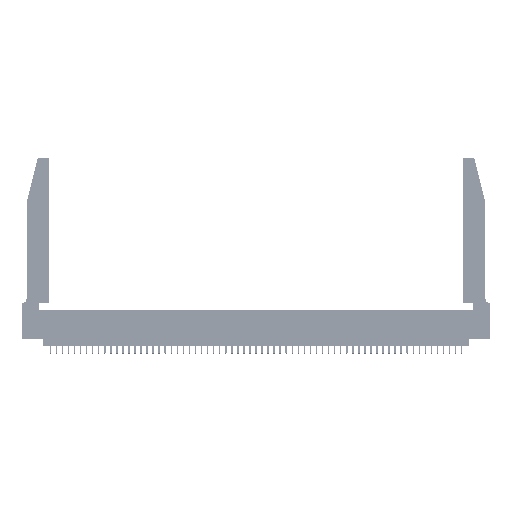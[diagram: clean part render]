
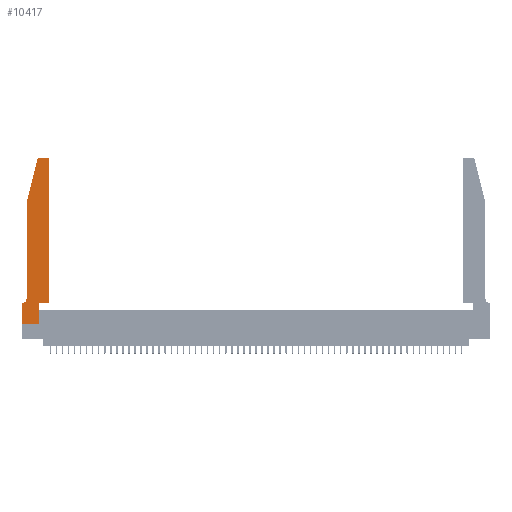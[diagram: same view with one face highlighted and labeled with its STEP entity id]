
A CAD part, top view. The second image highlights one B-rep face of the part: STEP entity #10417.
In plain terms, the highlighted planar face has unit normal (0, 0, 1).
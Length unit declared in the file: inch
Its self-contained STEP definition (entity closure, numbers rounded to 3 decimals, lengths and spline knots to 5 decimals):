
#891 = PLANE ( 'NONE',  #10989 ) ;
#2058 = EDGE_CURVE ( 'NONE', #8931, #30451, #37048, .T. ) ;
#2872 = DIRECTION ( 'NONE',  ( 0., 1., 0. ) ) ;
#3348 = ORIENTED_EDGE ( 'NONE', *, *, #26619, .T. ) ;
#3989 = CARTESIAN_POINT ( 'NONE',  ( 0.4205, 2.75, 0.37 ) ) ;
#4264 = AXIS2_PLACEMENT_3D ( 'NONE', #21716, #38909, #36018 ) ;
#4427 = EDGE_CURVE ( 'NONE', #45194, #24792, #38880, .T. ) ;
#4433 = VECTOR ( 'NONE', #43023, 39.37008 ) ;
#4806 = DIRECTION ( 'NONE',  ( 0., 0., 1. ) ) ;
#4918 = CARTESIAN_POINT ( 'NONE',  ( 0.4505, 0.35, 0.37 ) ) ;
#6414 = ORIENTED_EDGE ( 'NONE', *, *, #10900, .T. ) ;
#8605 = CARTESIAN_POINT ( 'NONE',  ( 0., 0.35, 0.37 ) ) ;
#8931 = VERTEX_POINT ( 'NONE', #50287 ) ;
#9061 = EDGE_CURVE ( 'NONE', #31428, #45194, #43631, .T. ) ;
#9424 = CARTESIAN_POINT ( 'NONE',  ( 0.4505, 0.35, 0.37 ) ) ;
#10417 = ADVANCED_FACE ( 'NONE', ( #13896 ), #891, .T. ) ;
#10900 = EDGE_CURVE ( 'NONE', #27365, #42193, #46105, .T. ) ;
#10989 = AXIS2_PLACEMENT_3D ( 'NONE', #25953, #4806, #17506 ) ;
#12014 = EDGE_CURVE ( 'NONE', #42193, #31428, #12374, .T. ) ;
#12374 = LINE ( 'NONE', #21118, #4433 ) ;
#12506 = LINE ( 'NONE', #4918, #15185 ) ;
#12856 = AXIS2_PLACEMENT_3D ( 'NONE', #47178, #42921, #17224 ) ;
#13137 = EDGE_CURVE ( 'NONE', #27929, #8931, #24853, .T. ) ;
#13896 = FACE_OUTER_BOUND ( 'NONE', #14380, .T. ) ;
#14380 = EDGE_LOOP ( 'NONE', ( #22211, #6414, #25425, #33420, #42155, #39651, #44276, #36805, #36044, #3348, #30424, #37566 ) ) ;
#14852 = VECTOR ( 'NONE', #47468, 39.37008 ) ;
#15185 = VECTOR ( 'NONE', #34869, 39.37008 ) ;
#17224 = DIRECTION ( 'NONE',  ( 1., 0., 0. ) ) ;
#17421 = CARTESIAN_POINT ( 'NONE',  ( 0.2865, 0.35, 0.37 ) ) ;
#17432 = LINE ( 'NONE', #52003, #25488 ) ;
#17506 = DIRECTION ( 'NONE',  ( 1., 0., 0. ) ) ;
#17520 = CARTESIAN_POINT ( 'NONE',  ( 0.2865, 0.35, 0.37 ) ) ;
#17792 = CARTESIAN_POINT ( 'NONE',  ( 0., 0., 0.37 ) ) ;
#18248 = EDGE_CURVE ( 'NONE', #48415, #41731, #26283, .T. ) ;
#19360 = CARTESIAN_POINT ( 'NONE',  ( 0.0755, 2., 0.37 ) ) ;
#21118 = CARTESIAN_POINT ( 'NONE',  ( 0.0755, 2., 0.37 ) ) ;
#21716 = CARTESIAN_POINT ( 'NONE',  ( 0.284, 2.72, 0.37 ) ) ;
#22126 = DIRECTION ( 'NONE',  ( 0., -1., 0. ) ) ;
#22211 = ORIENTED_EDGE ( 'NONE', *, *, #51842, .T. ) ;
#22424 = CARTESIAN_POINT ( 'NONE',  ( 0.284, 2.75, 0.37 ) ) ;
#23789 = DIRECTION ( 'NONE',  ( 0., 0., -1. ) ) ;
#23941 = DIRECTION ( 'NONE',  ( -1., 0., 0. ) ) ;
#24792 = VERTEX_POINT ( 'NONE', #25930 ) ;
#24811 = CARTESIAN_POINT ( 'NONE',  ( 0., 0., 0.37 ) ) ;
#24853 = LINE ( 'NONE', #50204, #46906 ) ;
#25425 = ORIENTED_EDGE ( 'NONE', *, *, #12014, .T. ) ;
#25488 = VECTOR ( 'NONE', #29948, 39.37008 ) ;
#25910 = DIRECTION ( 'NONE',  ( 0., -1., 0. ) ) ;
#25930 = CARTESIAN_POINT ( 'NONE',  ( 0.0055, 0.35, 0.37 ) ) ;
#25953 = CARTESIAN_POINT ( 'NONE',  ( 0., 0.35, 0.37 ) ) ;
#26283 = LINE ( 'NONE', #17520, #14852 ) ;
#26349 = CARTESIAN_POINT ( 'NONE',  ( 0.25487, 2.72718, 0.37 ) ) ;
#26619 = EDGE_CURVE ( 'NONE', #41731, #27929, #12506, .T. ) ;
#26901 = CARTESIAN_POINT ( 'NONE',  ( 0.0755, 0.42, 0.37 ) ) ;
#27365 = VERTEX_POINT ( 'NONE', #22424 ) ;
#27472 = CARTESIAN_POINT ( 'NONE',  ( 0.2605, 2.75, 0.37 ) ) ;
#27929 = VERTEX_POINT ( 'NONE', #9424 ) ;
#28119 = VECTOR ( 'NONE', #54023, 39.37008 ) ;
#29222 = VERTEX_POINT ( 'NONE', #8605 ) ;
#29918 = VERTEX_POINT ( 'NONE', #47608 ) ;
#29948 = DIRECTION ( 'NONE',  ( -1., 0., 0. ) ) ;
#30424 = ORIENTED_EDGE ( 'NONE', *, *, #13137, .T. ) ;
#30451 = VERTEX_POINT ( 'NONE', #3989 ) ;
#31428 = VERTEX_POINT ( 'NONE', #19360 ) ;
#33420 = ORIENTED_EDGE ( 'NONE', *, *, #9061, .T. ) ;
#34869 = DIRECTION ( 'NONE',  ( 1., 0., 0. ) ) ;
#36018 = DIRECTION ( 'NONE',  ( 1., 0., 0. ) ) ;
#36044 = ORIENTED_EDGE ( 'NONE', *, *, #18248, .T. ) ;
#36700 = DIRECTION ( 'NONE',  ( -1., 0., 0. ) ) ;
#36805 = ORIENTED_EDGE ( 'NONE', *, *, #37416, .T. ) ;
#37048 = CIRCLE ( 'NONE', #12856, 0.03 ) ;
#37416 = EDGE_CURVE ( 'NONE', #29918, #48415, #51623, .T. ) ;
#37566 = ORIENTED_EDGE ( 'NONE', *, *, #2058, .T. ) ;
#38515 = VECTOR ( 'NONE', #22126, 39.37008 ) ;
#38880 = CIRCLE ( 'NONE', #51717, 0.07 ) ;
#38909 = DIRECTION ( 'NONE',  ( 0., 0., 1. ) ) ;
#39651 = ORIENTED_EDGE ( 'NONE', *, *, #55420, .T. ) ;
#41731 = VERTEX_POINT ( 'NONE', #17421 ) ;
#41793 = LINE ( 'NONE', #27472, #43752 ) ;
#42155 = ORIENTED_EDGE ( 'NONE', *, *, #4427, .T. ) ;
#42193 = VERTEX_POINT ( 'NONE', #26349 ) ;
#42921 = DIRECTION ( 'NONE',  ( 0., 0., 1. ) ) ;
#43023 = DIRECTION ( 'NONE',  ( -0.239, -0.971, 0. ) ) ;
#43631 = LINE ( 'NONE', #46887, #45604 ) ;
#43752 = VECTOR ( 'NONE', #23941, 39.37008 ) ;
#44276 = ORIENTED_EDGE ( 'NONE', *, *, #51175, .T. ) ;
#45194 = VERTEX_POINT ( 'NONE', #26901 ) ;
#45604 = VECTOR ( 'NONE', #25910, 39.37008 ) ;
#46105 = CIRCLE ( 'NONE', #4264, 0.03 ) ;
#46887 = CARTESIAN_POINT ( 'NONE',  ( 0.0755, 2., 0.37 ) ) ;
#46906 = VECTOR ( 'NONE', #2872, 39.37008 ) ;
#47178 = CARTESIAN_POINT ( 'NONE',  ( 0.4205, 2.72, 0.37 ) ) ;
#47468 = DIRECTION ( 'NONE',  ( 0., 1., 0. ) ) ;
#47608 = CARTESIAN_POINT ( 'NONE',  ( 0., 0., 0.37 ) ) ;
#48415 = VERTEX_POINT ( 'NONE', #52129 ) ;
#49411 = CARTESIAN_POINT ( 'NONE',  ( 0.0055, 0.42, 0.37 ) ) ;
#49867 = LINE ( 'NONE', #17792, #38515 ) ;
#50204 = CARTESIAN_POINT ( 'NONE',  ( 0.4505, 0.35, 0.37 ) ) ;
#50287 = CARTESIAN_POINT ( 'NONE',  ( 0.4505, 2.72, 0.37 ) ) ;
#51175 = EDGE_CURVE ( 'NONE', #29222, #29918, #49867, .T. ) ;
#51623 = LINE ( 'NONE', #24811, #28119 ) ;
#51717 = AXIS2_PLACEMENT_3D ( 'NONE', #49411, #23789, #36700 ) ;
#51842 = EDGE_CURVE ( 'NONE', #30451, #27365, #41793, .T. ) ;
#52003 = CARTESIAN_POINT ( 'NONE',  ( 0.0755, 0.35, 0.37 ) ) ;
#52129 = CARTESIAN_POINT ( 'NONE',  ( 0.2865, 0., 0.37 ) ) ;
#54023 = DIRECTION ( 'NONE',  ( 1., 0., 0. ) ) ;
#55420 = EDGE_CURVE ( 'NONE', #24792, #29222, #17432, .T. ) ;
